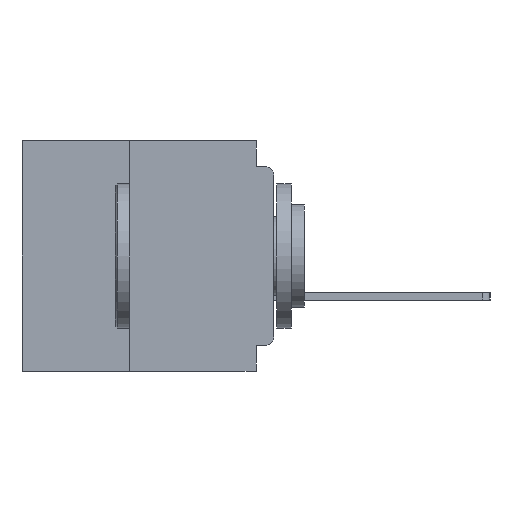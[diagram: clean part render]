
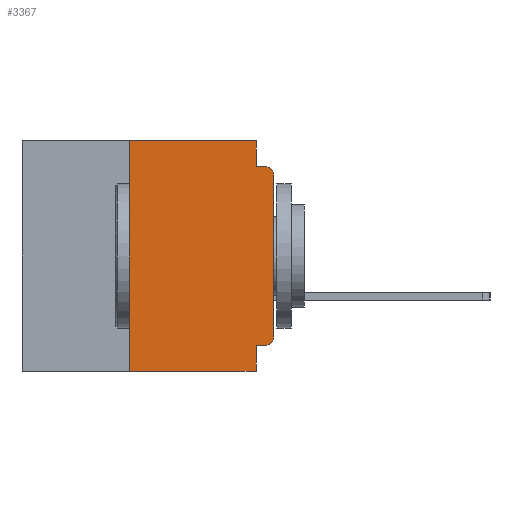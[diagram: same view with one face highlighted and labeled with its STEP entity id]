
A CAD part, left-side view. The second image highlights one B-rep face of the part: STEP entity #3367.
In plain terms, the highlighted planar face has unit normal (-1, 0, 0).
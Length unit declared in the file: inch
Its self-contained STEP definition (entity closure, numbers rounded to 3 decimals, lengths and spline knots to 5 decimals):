
#175 = CIRCLE ( 'NONE', #64684, 0.015 ) ;
#211 = VERTEX_POINT ( 'NONE', #4300 ) ;
#1695 = ORIENTED_EDGE ( 'NONE', *, *, #40643, .T. ) ;
#3102 = EDGE_CURVE ( 'NONE', #34656, #6088, #37206, .T. ) ;
#3367 = ADVANCED_FACE ( 'NONE', ( #8763 ), #9339, .F. ) ;
#4241 = CARTESIAN_POINT ( 'NONE',  ( 0., 0., -0.06 ) ) ;
#4300 = CARTESIAN_POINT ( 'NONE',  ( 0., 0., -0.34 ) ) ;
#4953 = VERTEX_POINT ( 'NONE', #42002 ) ;
#5670 = VERTEX_POINT ( 'NONE', #11768 ) ;
#6088 = VERTEX_POINT ( 'NONE', #41179 ) ;
#6850 = CIRCLE ( 'NONE', #7465, 0.015 ) ;
#7465 = AXIS2_PLACEMENT_3D ( 'NONE', #52287, #21224, #57475 ) ;
#7608 = EDGE_CURVE ( 'NONE', #21459, #4953, #24432, .T. ) ;
#8710 = ORIENTED_EDGE ( 'NONE', *, *, #40627, .F. ) ;
#8763 = FACE_OUTER_BOUND ( 'NONE', #50008, .T. ) ;
#9120 = DIRECTION ( 'NONE',  ( 0., 0., 1. ) ) ;
#9339 = PLANE ( 'NONE',  #43161 ) ;
#9693 = ORIENTED_EDGE ( 'NONE', *, *, #29866, .T. ) ;
#10080 = DIRECTION ( 'NONE',  ( 0., 0., 1. ) ) ;
#11768 = CARTESIAN_POINT ( 'NONE',  ( 0., 0.015, -0.355 ) ) ;
#13072 = DIRECTION ( 'NONE',  ( 0., -1., 0. ) ) ;
#13986 = ORIENTED_EDGE ( 'NONE', *, *, #7608, .F. ) ;
#14281 = VERTEX_POINT ( 'NONE', #54777 ) ;
#14383 = DIRECTION ( 'NONE',  ( 0., 0., -1. ) ) ;
#14571 = DIRECTION ( 'NONE',  ( 1., 0., 0. ) ) ;
#16260 = VECTOR ( 'NONE', #56449, 39.37008 ) ;
#21224 = DIRECTION ( 'NONE',  ( -1., 0., 0. ) ) ;
#21459 = VERTEX_POINT ( 'NONE', #34381 ) ;
#21739 = EDGE_CURVE ( 'NONE', #63824, #21459, #37135, .T. ) ;
#23292 = VECTOR ( 'NONE', #14383, 39.37008 ) ;
#24042 = VECTOR ( 'NONE', #13072, 39.37008 ) ;
#24432 = LINE ( 'NONE', #56103, #65772 ) ;
#24534 = CARTESIAN_POINT ( 'NONE',  ( 0., 0.031, 0. ) ) ;
#25288 = VECTOR ( 'NONE', #10080, 39.37008 ) ;
#26198 = VECTOR ( 'NONE', #9120, 39.37008 ) ;
#26386 = EDGE_CURVE ( 'NONE', #57052, #6088, #30055, .T. ) ;
#26880 = ORIENTED_EDGE ( 'NONE', *, *, #52720, .T. ) ;
#27465 = CARTESIAN_POINT ( 'NONE',  ( 0., 0.031, -0.355 ) ) ;
#28484 = CARTESIAN_POINT ( 'NONE',  ( 0., 0.437, 0. ) ) ;
#29866 = EDGE_CURVE ( 'NONE', #211, #51342, #30194, .T. ) ;
#29985 = CARTESIAN_POINT ( 'NONE',  ( 0., 0.015, -0.06 ) ) ;
#30055 = LINE ( 'NONE', #46068, #16260 ) ;
#30194 = LINE ( 'NONE', #46358, #25288 ) ;
#30425 = CARTESIAN_POINT ( 'NONE',  ( 0., 0., -0.355 ) ) ;
#32753 = CARTESIAN_POINT ( 'NONE',  ( 0., 0.437, -0.4 ) ) ;
#33500 = VECTOR ( 'NONE', #56446, 39.37008 ) ;
#34381 = CARTESIAN_POINT ( 'NONE',  ( 0., 0.031, -0.045 ) ) ;
#34656 = VERTEX_POINT ( 'NONE', #54688 ) ;
#35221 = DIRECTION ( 'NONE',  ( 0., 0., -1. ) ) ;
#35513 = CARTESIAN_POINT ( 'NONE',  ( 0., 0.031, 0. ) ) ;
#36206 = ORIENTED_EDGE ( 'NONE', *, *, #48647, .F. ) ;
#36762 = LINE ( 'NONE', #30425, #33500 ) ;
#37135 = LINE ( 'NONE', #24534, #23292 ) ;
#37206 = LINE ( 'NONE', #32753, #63092 ) ;
#39410 = ORIENTED_EDGE ( 'NONE', *, *, #26386, .F. ) ;
#40411 = CARTESIAN_POINT ( 'NONE',  ( 0., 0.437, 0. ) ) ;
#40627 = EDGE_CURVE ( 'NONE', #34656, #14281, #55397, .T. ) ;
#40643 = EDGE_CURVE ( 'NONE', #51342, #4953, #175, .T. ) ;
#40722 = EDGE_CURVE ( 'NONE', #5670, #57052, #36762, .T. ) ;
#41179 = CARTESIAN_POINT ( 'NONE',  ( 0., 0.031, -0.4 ) ) ;
#42002 = CARTESIAN_POINT ( 'NONE',  ( 0., 0.015, -0.045 ) ) ;
#43161 = AXIS2_PLACEMENT_3D ( 'NONE', #40411, #14571, #50814 ) ;
#46068 = CARTESIAN_POINT ( 'NONE',  ( 0., 0.031, -0.4 ) ) ;
#46358 = CARTESIAN_POINT ( 'NONE',  ( 0., 0., 0. ) ) ;
#47956 = ORIENTED_EDGE ( 'NONE', *, *, #40722, .F. ) ;
#47973 = ORIENTED_EDGE ( 'NONE', *, *, #21739, .F. ) ;
#48647 = EDGE_CURVE ( 'NONE', #14281, #63824, #65378, .T. ) ;
#50008 = EDGE_LOOP ( 'NONE', ( #9693, #1695, #13986, #47973, #36206, #8710, #52472, #39410, #47956, #26880 ) ) ;
#50814 = DIRECTION ( 'NONE',  ( 0., 0., -1. ) ) ;
#50907 = DIRECTION ( 'NONE',  ( 0., -1., 0. ) ) ;
#51342 = VERTEX_POINT ( 'NONE', #4241 ) ;
#52287 = CARTESIAN_POINT ( 'NONE',  ( 0., 0.015, -0.34 ) ) ;
#52472 = ORIENTED_EDGE ( 'NONE', *, *, #3102, .T. ) ;
#52720 = EDGE_CURVE ( 'NONE', #5670, #211, #6850, .T. ) ;
#54688 = CARTESIAN_POINT ( 'NONE',  ( 0., 0.25, -0.4 ) ) ;
#54777 = CARTESIAN_POINT ( 'NONE',  ( 0., 0.25, 0. ) ) ;
#55397 = LINE ( 'NONE', #60769, #26198 ) ;
#56103 = CARTESIAN_POINT ( 'NONE',  ( 0., 0., -0.045 ) ) ;
#56446 = DIRECTION ( 'NONE',  ( 0., 1., 0. ) ) ;
#56449 = DIRECTION ( 'NONE',  ( 0., 0., -1. ) ) ;
#57052 = VERTEX_POINT ( 'NONE', #27465 ) ;
#57475 = DIRECTION ( 'NONE',  ( 0., 0., -1. ) ) ;
#60769 = CARTESIAN_POINT ( 'NONE',  ( 0., 0.25, -0.4 ) ) ;
#63092 = VECTOR ( 'NONE', #63956, 39.37008 ) ;
#63824 = VERTEX_POINT ( 'NONE', #35513 ) ;
#63956 = DIRECTION ( 'NONE',  ( 0., -1., 0. ) ) ;
#64684 = AXIS2_PLACEMENT_3D ( 'NONE', #29985, #66174, #35221 ) ;
#65378 = LINE ( 'NONE', #28484, #24042 ) ;
#65772 = VECTOR ( 'NONE', #50907, 39.37008 ) ;
#66174 = DIRECTION ( 'NONE',  ( -1., 0., 0. ) ) ;
